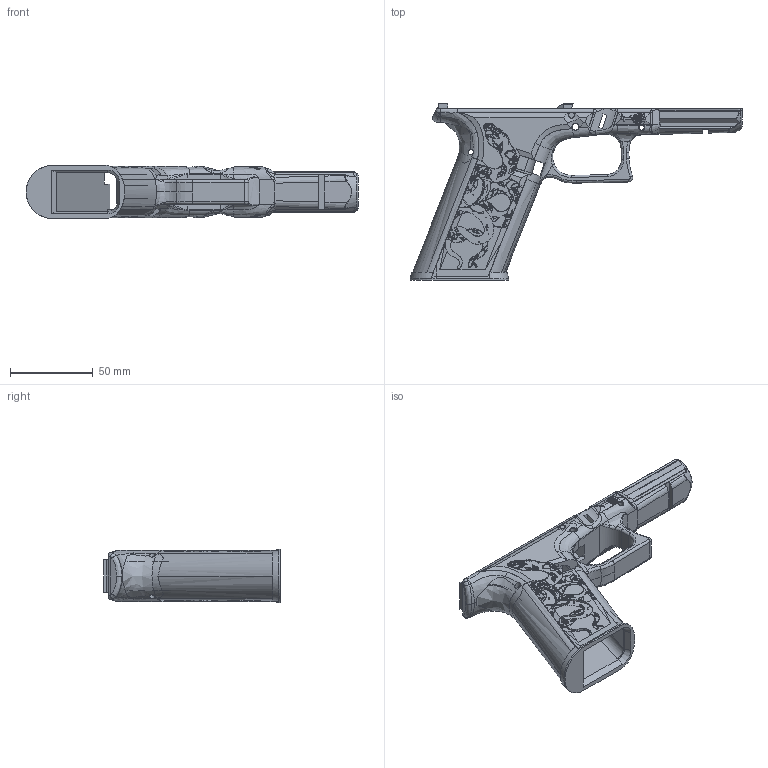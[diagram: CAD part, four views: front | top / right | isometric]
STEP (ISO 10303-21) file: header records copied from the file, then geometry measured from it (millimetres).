
FILE_DESCRIPTION(/* description */ (''),/* implementation_level */ '2;1');
FILE_NAME(/* name */ 'serpent.step',/* time_stamp */ '2021-09-01T23:43:24-04:00',/* author */ (''),/* organization */ (''),/* preprocessor_version */ 'ST-DEVELOPER v18.1',/* originating_system */ 'Autodesk Translation Framework v10.10.0.1391',/* authorisation */ '');
FILE_SCHEMA (('AUTOMOTIVE_DESIGN { 1 0 10303 214 3 1 1 }'));
Products named in the file (1): FMDA DD17.2 V1.4 Frame
Bounding box: 200 x 106.5 x 32 mm (x, y, z)
Volume: 93509.7 mm3; surface area: 51263 mm2
Topology: 1 solids, 3 shells, 5270 faces, 15162 edges, 10048 vertices
Faces by surface type: bspline 4538, plane 549, cylinder 123, cone 25, torus 19, sphere 16
Full cylindrical faces by diameter (mm): 2 x1, 3 x4, 3.2 x2, 4 x2
Entity records: 225134 total; most frequent: CARTESIAN_POINT 127597, ORIENTED_EDGE 30306, EDGE_CURVE 15153, VERTEX_POINT 10048, DIRECTION 7688, EDGE_LOOP 5459, FACE_OUTER_BOUND 5270, ADVANCED_FACE 5270
